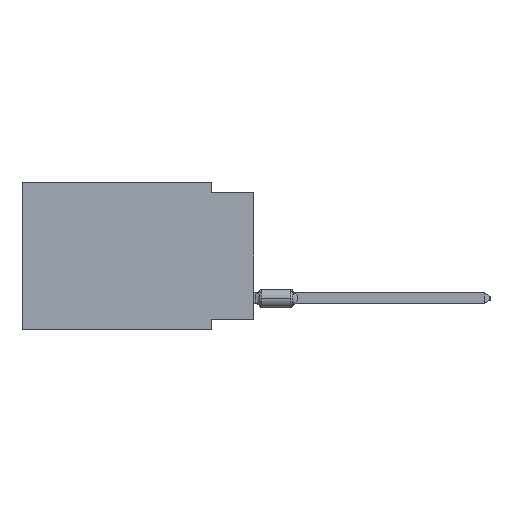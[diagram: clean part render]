
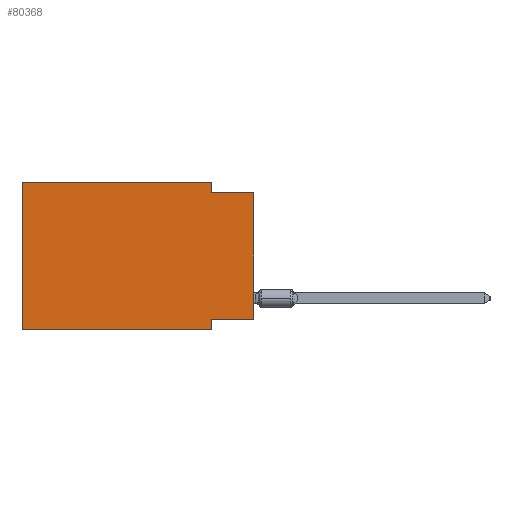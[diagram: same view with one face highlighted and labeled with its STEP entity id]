
A CAD part, left-side view. The second image highlights one B-rep face of the part: STEP entity #80368.
In plain terms, the highlighted planar face has unit normal (-1, 0, 0).
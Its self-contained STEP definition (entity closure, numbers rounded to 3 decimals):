
#533 = VERTEX_POINT ( 'NONE', #44989 ) ;
#1177 = CARTESIAN_POINT ( 'NONE',  ( 0., 2.54, -8.255 ) ) ;
#2233 = EDGE_CURVE ( 'NONE', #65799, #533, #74076, .T. ) ;
#3875 = DIRECTION ( 'NONE',  ( 0., -1., 0. ) ) ;
#4278 = VERTEX_POINT ( 'NONE', #41292 ) ;
#7262 = EDGE_CURVE ( 'NONE', #533, #4278, #88142, .T. ) ;
#7744 = VECTOR ( 'NONE', #72878, 1000. ) ;
#9905 = VECTOR ( 'NONE', #51520, 1000. ) ;
#12405 = VERTEX_POINT ( 'NONE', #1177 ) ;
#15885 = LINE ( 'NONE', #80117, #70514 ) ;
#16382 = EDGE_CURVE ( 'NONE', #58821, #12405, #88482, .T. ) ;
#17196 = EDGE_CURVE ( 'NONE', #68141, #65799, #82960, .T. ) ;
#19011 = CARTESIAN_POINT ( 'NONE',  ( 0., 2.54, -8.89 ) ) ;
#19616 = ORIENTED_EDGE ( 'NONE', *, *, #16382, .F. ) ;
#20873 = CARTESIAN_POINT ( 'NONE',  ( 0., 0., -8.255 ) ) ;
#21118 = ORIENTED_EDGE ( 'NONE', *, *, #7262, .F. ) ;
#23518 = VERTEX_POINT ( 'NONE', #70151 ) ;
#28436 = ORIENTED_EDGE ( 'NONE', *, *, #2233, .F. ) ;
#30306 = DIRECTION ( 'NONE',  ( 0., -1., 0. ) ) ;
#31473 = CARTESIAN_POINT ( 'NONE',  ( 0., 13.97, -8.89 ) ) ;
#32146 = CARTESIAN_POINT ( 'NONE',  ( 0., 0., -8.255 ) ) ;
#32300 = PLANE ( 'NONE',  #84573 ) ;
#36332 = EDGE_CURVE ( 'NONE', #58821, #4278, #89469, .T. ) ;
#37749 = VECTOR ( 'NONE', #3875, 1000. ) ;
#40978 = ORIENTED_EDGE ( 'NONE', *, *, #17196, .F. ) ;
#41292 = CARTESIAN_POINT ( 'NONE',  ( 0., 0., -0.635 ) ) ;
#43077 = VERTEX_POINT ( 'NONE', #31473 ) ;
#43191 = VECTOR ( 'NONE', #48532, 1000. ) ;
#44487 = ORIENTED_EDGE ( 'NONE', *, *, #84464, .F. ) ;
#44989 = CARTESIAN_POINT ( 'NONE',  ( 0., 2.54, -0.635 ) ) ;
#44995 = CARTESIAN_POINT ( 'NONE',  ( 0., 13.97, 0. ) ) ;
#45388 = CARTESIAN_POINT ( 'NONE',  ( 0., 13.97, 0. ) ) ;
#46138 = DIRECTION ( 'NONE',  ( 0., 1., 0. ) ) ;
#47409 = DIRECTION ( 'NONE',  ( 0., 0., -1. ) ) ;
#48532 = DIRECTION ( 'NONE',  ( 0., -1., 0. ) ) ;
#49893 = EDGE_CURVE ( 'NONE', #43077, #23518, #15885, .T. ) ;
#51520 = DIRECTION ( 'NONE',  ( 0., 0., 1. ) ) ;
#52697 = CARTESIAN_POINT ( 'NONE',  ( 0., 2.54, 0. ) ) ;
#53389 = ORIENTED_EDGE ( 'NONE', *, *, #68654, .F. ) ;
#54108 = CARTESIAN_POINT ( 'NONE',  ( 0., 0., 0. ) ) ;
#58821 = VERTEX_POINT ( 'NONE', #20873 ) ;
#60111 = DIRECTION ( 'NONE',  ( 0., 0., -1. ) ) ;
#60234 = DIRECTION ( 'NONE',  ( 1., 0., 0. ) ) ;
#64319 = VECTOR ( 'NONE', #47409, 1000. ) ;
#65799 = VERTEX_POINT ( 'NONE', #78741 ) ;
#65930 = LINE ( 'NONE', #44995, #9905 ) ;
#68141 = VERTEX_POINT ( 'NONE', #78605 ) ;
#68654 = EDGE_CURVE ( 'NONE', #43077, #68141, #65930, .T. ) ;
#70151 = CARTESIAN_POINT ( 'NONE',  ( 0., 2.54, -8.89 ) ) ;
#70514 = VECTOR ( 'NONE', #30306, 1000. ) ;
#71722 = ORIENTED_EDGE ( 'NONE', *, *, #36332, .T. ) ;
#72878 = DIRECTION ( 'NONE',  ( 0., 0., 1. ) ) ;
#73297 = ORIENTED_EDGE ( 'NONE', *, *, #49893, .T. ) ;
#73298 = FACE_OUTER_BOUND ( 'NONE', #79381, .T. ) ;
#74076 = LINE ( 'NONE', #52697, #84470 ) ;
#74657 = DIRECTION ( 'NONE',  ( 0., 0., -1. ) ) ;
#75971 = CARTESIAN_POINT ( 'NONE',  ( 0., 13.97, 0. ) ) ;
#78605 = CARTESIAN_POINT ( 'NONE',  ( 0., 13.97, 0. ) ) ;
#78741 = CARTESIAN_POINT ( 'NONE',  ( 0., 2.54, 0. ) ) ;
#79381 = EDGE_LOOP ( 'NONE', ( #71722, #21118, #28436, #40978, #53389, #73297, #44487, #19616 ) ) ;
#80117 = CARTESIAN_POINT ( 'NONE',  ( 0., 13.97, -8.89 ) ) ;
#80278 = VECTOR ( 'NONE', #46138, 1000. ) ;
#80368 = ADVANCED_FACE ( 'NONE', ( #73298 ), #32300, .F. ) ;
#82960 = LINE ( 'NONE', #75971, #43191 ) ;
#84464 = EDGE_CURVE ( 'NONE', #12405, #23518, #89283, .T. ) ;
#84470 = VECTOR ( 'NONE', #60111, 1000. ) ;
#84573 = AXIS2_PLACEMENT_3D ( 'NONE', #45388, #60234, #74657 ) ;
#88142 = LINE ( 'NONE', #88592, #37749 ) ;
#88482 = LINE ( 'NONE', #32146, #80278 ) ;
#88592 = CARTESIAN_POINT ( 'NONE',  ( 0., 0., -0.635 ) ) ;
#89283 = LINE ( 'NONE', #19011, #64319 ) ;
#89469 = LINE ( 'NONE', #54108, #7744 ) ;
